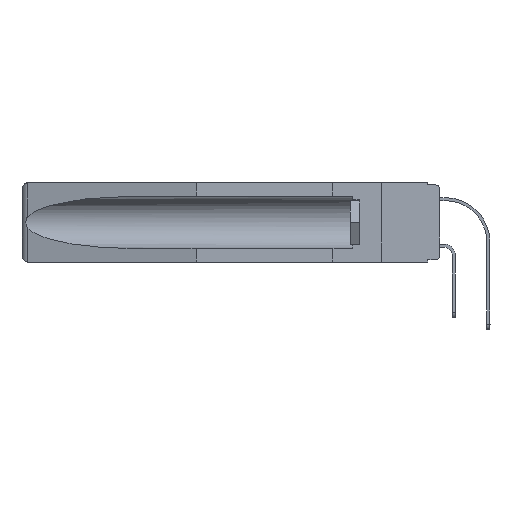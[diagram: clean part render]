
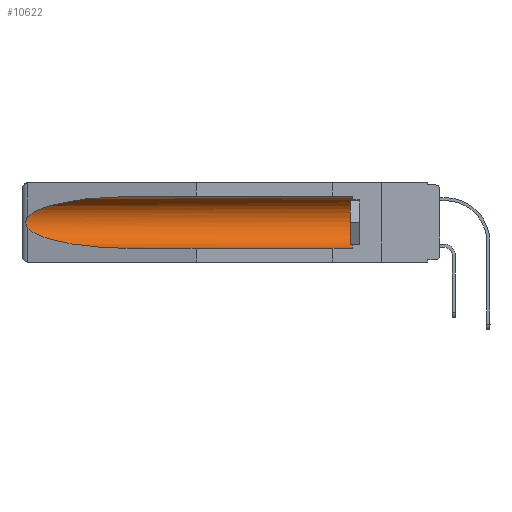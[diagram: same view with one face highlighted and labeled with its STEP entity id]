
A CAD part, left-side view. The second image highlights one B-rep face of the part: STEP entity #10622.
In plain terms, the highlighted cylindrical face has radius 2.857 mm (diameter 5.715 mm), a partial arc.
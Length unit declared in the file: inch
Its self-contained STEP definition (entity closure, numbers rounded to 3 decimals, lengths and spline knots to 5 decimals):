
#1639 = CARTESIAN_POINT ( 'NONE',  ( 0.2675, 1.53308, -0.16763 ) ) ;
#1745 = CARTESIAN_POINT ( 'NONE',  ( 0.26537, 1.52718, -0.14972 ) ) ;
#2776 = CARTESIAN_POINT ( 'NONE',  ( 0.25451, 1.48313, -0.24835 ) ) ;
#3128 = CARTESIAN_POINT ( 'NONE',  ( 0.26537, 1.52718, -0.19328 ) ) ;
#3369 = ORIENTED_EDGE ( 'NONE', *, *, #22153, .T. ) ;
#3550 = FACE_OUTER_BOUND ( 'NONE', #3756, .T. ) ;
#3756 = EDGE_LOOP ( 'NONE', ( #15613, #11478, #3369, #4724, #21409, #19275 ) ) ;
#4554 = EDGE_CURVE ( 'NONE', #7757, #14989, #19396, .T. ) ;
#4724 = ORIENTED_EDGE ( 'NONE', *, *, #14915, .F. ) ;
#4873 = CARTESIAN_POINT ( 'NONE',  ( 0.25451, 1.48313, -0.09465 ) ) ;
#5403 = DIRECTION ( 'NONE',  ( 0., 0., 1. ) ) ;
#6130 = CARTESIAN_POINT ( 'NONE',  ( 0.21114, 1.30732, -0.284 ) ) ;
#6220 = VERTEX_POINT ( 'NONE', #18948 ) ;
#6480 = CARTESIAN_POINT ( 'NONE',  ( 0.155, 1.07973, -0.059 ) ) ;
#6710 = CARTESIAN_POINT ( 'NONE',  ( 0.26654, 1.53092, -0.15636 ) ) ;
#6875 = CARTESIAN_POINT ( 'NONE',  ( 0.155, -0.30754, -0.059 ) ) ;
#7500 = CARTESIAN_POINT ( 'NONE',  ( 0.26537, 1.52718, -0.19328 ) ) ;
#7757 = VERTEX_POINT ( 'NONE', #22001 ) ;
#8095 = CARTESIAN_POINT ( 'NONE',  ( 0.155, 1.07973, -0.284 ) ) ;
#8394 = CARTESIAN_POINT ( 'NONE',  ( 0.155, 0.126, -0.1715 ) ) ;
#8669 = CARTESIAN_POINT ( 'NONE',  ( 0.2675, 1.53308, -0.17534 ) ) ;
#9251 = CARTESIAN_POINT ( 'NONE',  ( 0.155, -0.30754, -0.284 ) ) ;
#9371 = EDGE_CURVE ( 'NONE', #11863, #14947, #12996, .T. ) ;
#9948 = CARTESIAN_POINT ( 'NONE',  ( 0.26537, 1.52718, -0.19328 ) ) ;
#10241 = DIRECTION ( 'NONE',  ( 0., 1., 0. ) ) ;
#10300 = CARTESIAN_POINT ( 'NONE',  ( 0.26655, 1.53094, -0.18657 ) ) ;
#10610 = CYLINDRICAL_SURFACE ( 'NONE', #20994, 0.1125 ) ;
#10622 = ADVANCED_FACE ( 'NONE', ( #3550 ), #10610, .F. ) ;
#11100 =( BOUNDED_CURVE ( )  B_SPLINE_CURVE ( 3, ( #9948, #2776, #6130, #8095 ),
 .UNSPECIFIED., .F., .F. ) 
 B_SPLINE_CURVE_WITH_KNOTS ( ( 4, 4 ),
 ( 0.1948, 1.5708 ),
 .UNSPECIFIED. ) 
 CURVE ( )  GEOMETRIC_REPRESENTATION_ITEM ( )  RATIONAL_B_SPLINE_CURVE ( ( 1., 0.848, 0.848, 1. ) ) 
 REPRESENTATION_ITEM ( '' )  );
#11478 = ORIENTED_EDGE ( 'NONE', *, *, #9371, .T. ) ;
#11777 = VECTOR ( 'NONE', #16675, 39.37008 ) ;
#11863 = VERTEX_POINT ( 'NONE', #19583 ) ;
#12152 = EDGE_CURVE ( 'NONE', #14989, #6220, #22785, .T. ) ;
#12168 = CARTESIAN_POINT ( 'NONE',  ( 0.21114, 1.30732, -0.059 ) ) ;
#12343 = AXIS2_PLACEMENT_3D ( 'NONE', #8394, #15473, #22562 ) ;
#12595 = CARTESIAN_POINT ( 'NONE',  ( 0.155, -0.30754, -0.1715 ) ) ;
#12996 = B_SPLINE_CURVE_WITH_KNOTS ( 'NONE', 3,
 ( #1745, #22612, #6710, #15295, #1639, #8669, #19372, #10300, #22373, #3128 ),
 .UNSPECIFIED., .F., .F.,
 ( 4, 2, 2, 2, 4 ),
 ( 0., 0.00029, 0.00058, 0.00087, 0.00117 ),
 .UNSPECIFIED. ) ;
#14582 = LINE ( 'NONE', #9251, #11777 ) ;
#14915 = EDGE_CURVE ( 'NONE', #7757, #22731, #14582, .T. ) ;
#14947 = VERTEX_POINT ( 'NONE', #7500 ) ;
#14989 = VERTEX_POINT ( 'NONE', #19933 ) ;
#15295 = CARTESIAN_POINT ( 'NONE',  ( 0.2673, 1.5327, -0.16383 ) ) ;
#15473 = DIRECTION ( 'NONE',  ( 0., -1., 0. ) ) ;
#15613 = ORIENTED_EDGE ( 'NONE', *, *, #17292, .T. ) ;
#16035 = CARTESIAN_POINT ( 'NONE',  ( 0.155, 1.07973, -0.284 ) ) ;
#16675 = DIRECTION ( 'NONE',  ( 0., 1., 0. ) ) ;
#17292 = EDGE_CURVE ( 'NONE', #6220, #11863, #21487, .T. ) ;
#17706 = DIRECTION ( 'NONE',  ( 0., 1., 0. ) ) ;
#18790 = CARTESIAN_POINT ( 'NONE',  ( 0.26537, 1.52718, -0.14972 ) ) ;
#18948 = CARTESIAN_POINT ( 'NONE',  ( 0.155, 1.07973, -0.059 ) ) ;
#19275 = ORIENTED_EDGE ( 'NONE', *, *, #12152, .T. ) ;
#19372 = CARTESIAN_POINT ( 'NONE',  ( 0.2673, 1.53269, -0.17917 ) ) ;
#19396 = CIRCLE ( 'NONE', #12343, 0.1125 ) ;
#19583 = CARTESIAN_POINT ( 'NONE',  ( 0.26537, 1.52718, -0.14972 ) ) ;
#19587 = VECTOR ( 'NONE', #10241, 39.37008 ) ;
#19933 = CARTESIAN_POINT ( 'NONE',  ( 0.155, 0.126, -0.059 ) ) ;
#20994 = AXIS2_PLACEMENT_3D ( 'NONE', #12595, #17706, #5403 ) ;
#21409 = ORIENTED_EDGE ( 'NONE', *, *, #4554, .T. ) ;
#21487 =( BOUNDED_CURVE ( )  B_SPLINE_CURVE ( 3, ( #6480, #12168, #4873, #18790 ),
 .UNSPECIFIED., .F., .F. ) 
 B_SPLINE_CURVE_WITH_KNOTS ( ( 4, 4 ),
 ( 4.71239, 6.08839 ),
 .UNSPECIFIED. ) 
 CURVE ( )  GEOMETRIC_REPRESENTATION_ITEM ( )  RATIONAL_B_SPLINE_CURVE ( ( 1., 0.848, 0.848, 1. ) ) 
 REPRESENTATION_ITEM ( '' )  );
#22001 = CARTESIAN_POINT ( 'NONE',  ( 0.155, 0.126, -0.284 ) ) ;
#22153 = EDGE_CURVE ( 'NONE', #14947, #22731, #11100, .T. ) ;
#22373 = CARTESIAN_POINT ( 'NONE',  ( 0.26597, 1.5296, -0.19026 ) ) ;
#22562 = DIRECTION ( 'NONE',  ( 0., 0., 1. ) ) ;
#22612 = CARTESIAN_POINT ( 'NONE',  ( 0.26597, 1.52961, -0.15275 ) ) ;
#22731 = VERTEX_POINT ( 'NONE', #16035 ) ;
#22785 = LINE ( 'NONE', #6875, #19587 ) ;
